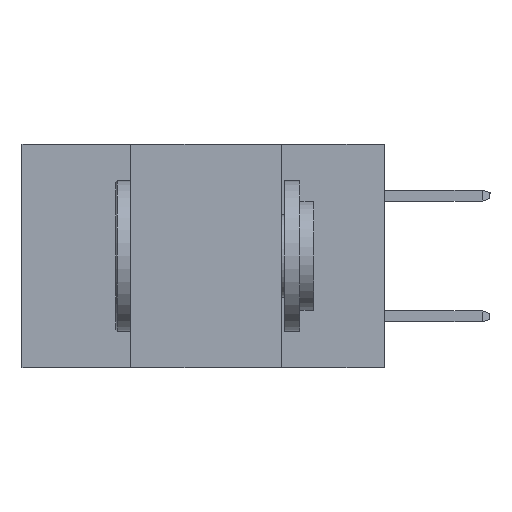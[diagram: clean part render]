
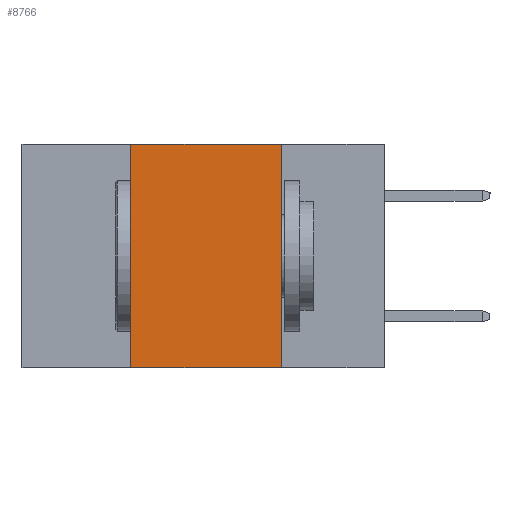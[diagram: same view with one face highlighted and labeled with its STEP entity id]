
A CAD part, left-side view. The second image highlights one B-rep face of the part: STEP entity #8766.
In plain terms, the highlighted planar face has unit normal (-1, 0, 0).
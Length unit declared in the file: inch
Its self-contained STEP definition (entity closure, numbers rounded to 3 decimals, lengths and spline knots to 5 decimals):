
#325 = AXIS2_PLACEMENT_3D ( 'NONE', #6594, #2764, #6891 ) ;
#465 = FACE_OUTER_BOUND ( 'NONE', #9042, .T. ) ;
#763 = EDGE_CURVE ( 'NONE', #4865, #7702, #6268, .T. ) ;
#912 = LINE ( 'NONE', #3871, #4270 ) ;
#934 = DIRECTION ( 'NONE',  ( 0., -1., 0. ) ) ;
#1120 = CARTESIAN_POINT ( 'NONE',  ( 0., 0.42, -0.37 ) ) ;
#2296 = DIRECTION ( 'NONE',  ( 0., 0., 1. ) ) ;
#2764 = DIRECTION ( 'NONE',  ( 1., 0., 0. ) ) ;
#3521 = PLANE ( 'NONE',  #325 ) ;
#3588 = EDGE_CURVE ( 'NONE', #4057, #7702, #6492, .T. ) ;
#3871 = CARTESIAN_POINT ( 'NONE',  ( 0., 0.6, 0. ) ) ;
#3968 = DIRECTION ( 'NONE',  ( 0., -1., 0. ) ) ;
#4057 = VERTEX_POINT ( 'NONE', #8926 ) ;
#4270 = VECTOR ( 'NONE', #3968, 39.37008 ) ;
#4865 = VERTEX_POINT ( 'NONE', #1120 ) ;
#5087 = EDGE_CURVE ( 'NONE', #7422, #4057, #912, .T. ) ;
#5098 = VECTOR ( 'NONE', #5757, 39.37008 ) ;
#5217 = ORIENTED_EDGE ( 'NONE', *, *, #3588, .F. ) ;
#5757 = DIRECTION ( 'NONE',  ( 0., 0., -1. ) ) ;
#6141 = CARTESIAN_POINT ( 'NONE',  ( 0., 0.42, -0.37 ) ) ;
#6268 = LINE ( 'NONE', #6314, #7639 ) ;
#6314 = CARTESIAN_POINT ( 'NONE',  ( 0., 0.6, -0.37 ) ) ;
#6492 = LINE ( 'NONE', #9559, #5098 ) ;
#6594 = CARTESIAN_POINT ( 'NONE',  ( 0., 0.6, 0. ) ) ;
#6872 = EDGE_CURVE ( 'NONE', #4865, #7422, #9187, .T. ) ;
#6891 = DIRECTION ( 'NONE',  ( 0., 0., -1. ) ) ;
#6898 = ORIENTED_EDGE ( 'NONE', *, *, #5087, .F. ) ;
#7422 = VERTEX_POINT ( 'NONE', #7687 ) ;
#7639 = VECTOR ( 'NONE', #934, 39.37008 ) ;
#7671 = VECTOR ( 'NONE', #2296, 39.37008 ) ;
#7687 = CARTESIAN_POINT ( 'NONE',  ( 0., 0.42, 0. ) ) ;
#7702 = VERTEX_POINT ( 'NONE', #9330 ) ;
#8253 = ORIENTED_EDGE ( 'NONE', *, *, #763, .T. ) ;
#8342 = ORIENTED_EDGE ( 'NONE', *, *, #6872, .F. ) ;
#8766 = ADVANCED_FACE ( 'NONE', ( #465 ), #3521, .F. ) ;
#8926 = CARTESIAN_POINT ( 'NONE',  ( 0., 0.17, 0. ) ) ;
#9042 = EDGE_LOOP ( 'NONE', ( #5217, #6898, #8342, #8253 ) ) ;
#9187 = LINE ( 'NONE', #6141, #7671 ) ;
#9330 = CARTESIAN_POINT ( 'NONE',  ( 0., 0.17, -0.37 ) ) ;
#9559 = CARTESIAN_POINT ( 'NONE',  ( 0., 0.17, -0.37 ) ) ;
